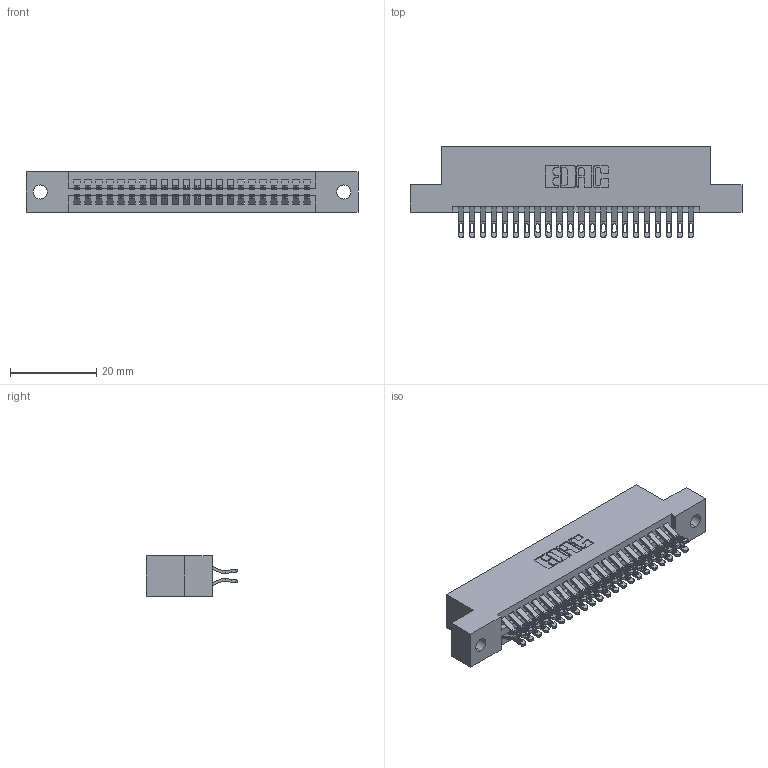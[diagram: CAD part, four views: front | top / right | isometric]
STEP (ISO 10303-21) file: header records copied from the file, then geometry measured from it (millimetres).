
FILE_DESCRIPTION (( 'STEP AP203' ), '1' );
FILE_NAME ('345-044-555-202.STEP', '2018-09-08T21:55:23', ( '' ), ( '' ), 'SwSTEP 2.0', 'SolidWorks 2016', '' );
FILE_SCHEMA (( 'CONFIG_CONTROL_DESIGN' ));
Length unit declared in the file: inch
Products named in the file (3): 345 Part_Flush Mounting Lugs - 0.128 Dia; 345-292-001_555 Tail; 345-044-555-202
Assembly tree (45 placements, depth 2):
  345-044-555-202
    345 Part_Flush Mounting Lugs - 0.128 Dia
    345-292-001_555 Tail  x44
Bounding box: 77.09 x 21.13 x 9.4 mm (x, y, z)
Volume: 7393.8 mm3; surface area: 10713.1 mm2
Topology: 45 solids, 45 shells, 2590 faces, 8129 edges, 5418 vertices
Faces by surface type: plane 1444, cylinder 1146
Entity records: 20283 total; most frequent: CARTESIAN_POINT 3454, ORIENTED_EDGE 3358, DIRECTION 3039, EDGE_CURVE 1679, LINE 1439, VECTOR 1439, VERTEX_POINT 1118, AXIS2_PLACEMENT_3D 800
